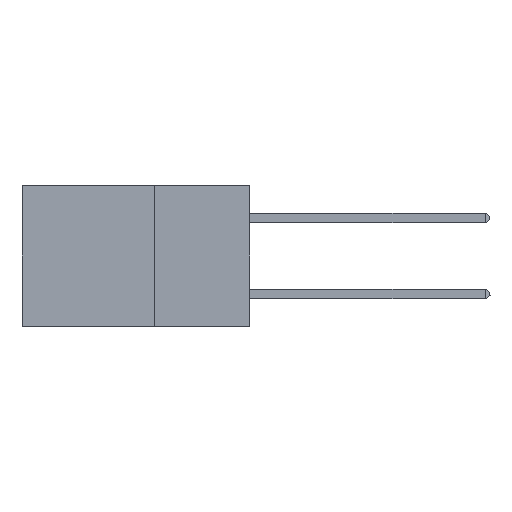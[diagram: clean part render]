
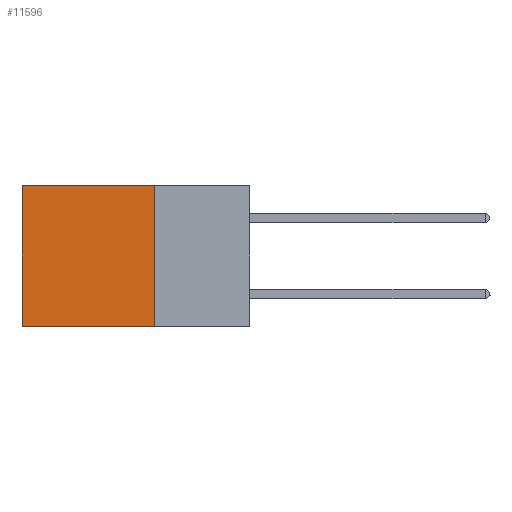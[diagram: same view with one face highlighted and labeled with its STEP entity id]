
A CAD part, left-side view. The second image highlights one B-rep face of the part: STEP entity #11596.
In plain terms, the highlighted planar face has unit normal (-1, 0, 0).
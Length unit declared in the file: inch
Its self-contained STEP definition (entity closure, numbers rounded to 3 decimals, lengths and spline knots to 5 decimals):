
#379 = EDGE_LOOP ( 'NONE', ( #17848, #12091, #19216, #20708 ) ) ;
#496 = LINE ( 'NONE', #22889, #15067 ) ;
#1358 = CARTESIAN_POINT ( 'NONE',  ( 0.2875, 0.6, -0.37 ) ) ;
#2008 = VECTOR ( 'NONE', #28170, 39.37008 ) ;
#2164 = LINE ( 'NONE', #22062, #25537 ) ;
#3915 = CARTESIAN_POINT ( 'NONE',  ( 0.2875, 0.25, -0.37 ) ) ;
#6143 = EDGE_CURVE ( 'NONE', #10917, #21111, #10819, .T. ) ;
#6281 = VECTOR ( 'NONE', #7732, 39.37008 ) ;
#6305 = DIRECTION ( 'NONE',  ( 0., 0., -1. ) ) ;
#7636 = CARTESIAN_POINT ( 'NONE',  ( 0.2875, 0.25, 0. ) ) ;
#7732 = DIRECTION ( 'NONE',  ( 0., 1., 0. ) ) ;
#10819 = LINE ( 'NONE', #7636, #6281 ) ;
#10917 = VERTEX_POINT ( 'NONE', #16921 ) ;
#11048 = EDGE_CURVE ( 'NONE', #10917, #20724, #496, .T. ) ;
#11357 = AXIS2_PLACEMENT_3D ( 'NONE', #22140, #22756, #6305 ) ;
#11596 = ADVANCED_FACE ( 'NONE', ( #26172 ), #23569, .F. ) ;
#12091 = ORIENTED_EDGE ( 'NONE', *, *, #31002, .F. ) ;
#12283 = DIRECTION ( 'NONE',  ( 0., 0., -1. ) ) ;
#15067 = VECTOR ( 'NONE', #20290, 39.37008 ) ;
#16921 = CARTESIAN_POINT ( 'NONE',  ( 0.2875, 0.25, 0. ) ) ;
#17591 = VERTEX_POINT ( 'NONE', #1358 ) ;
#17689 = LINE ( 'NONE', #23400, #2008 ) ;
#17848 = ORIENTED_EDGE ( 'NONE', *, *, #28376, .T. ) ;
#19216 = ORIENTED_EDGE ( 'NONE', *, *, #11048, .F. ) ;
#20290 = DIRECTION ( 'NONE',  ( 0., 0., -1. ) ) ;
#20708 = ORIENTED_EDGE ( 'NONE', *, *, #6143, .T. ) ;
#20724 = VERTEX_POINT ( 'NONE', #3915 ) ;
#21111 = VERTEX_POINT ( 'NONE', #29636 ) ;
#22062 = CARTESIAN_POINT ( 'NONE',  ( 0.2875, 0.6, 0. ) ) ;
#22140 = CARTESIAN_POINT ( 'NONE',  ( 0.2875, 0.25, 0. ) ) ;
#22756 = DIRECTION ( 'NONE',  ( 1., 0., 0. ) ) ;
#22889 = CARTESIAN_POINT ( 'NONE',  ( 0.2875, 0.25, 0. ) ) ;
#23400 = CARTESIAN_POINT ( 'NONE',  ( 0.2875, 0.25, -0.37 ) ) ;
#23569 = PLANE ( 'NONE',  #11357 ) ;
#25537 = VECTOR ( 'NONE', #12283, 39.37008 ) ;
#26172 = FACE_OUTER_BOUND ( 'NONE', #379, .T. ) ;
#28170 = DIRECTION ( 'NONE',  ( 0., 1., 0. ) ) ;
#28376 = EDGE_CURVE ( 'NONE', #21111, #17591, #2164, .T. ) ;
#29636 = CARTESIAN_POINT ( 'NONE',  ( 0.2875, 0.6, 0. ) ) ;
#31002 = EDGE_CURVE ( 'NONE', #20724, #17591, #17689, .T. ) ;
